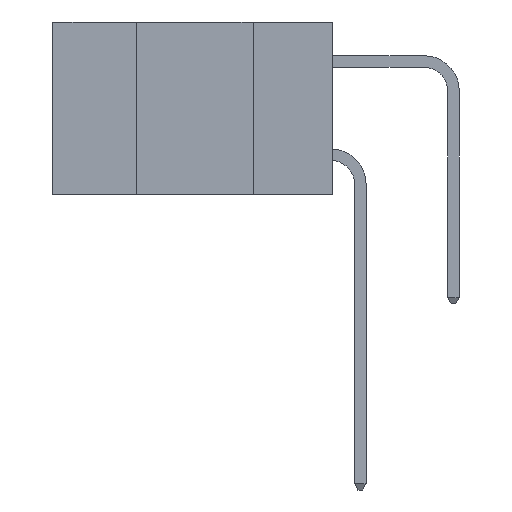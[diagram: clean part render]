
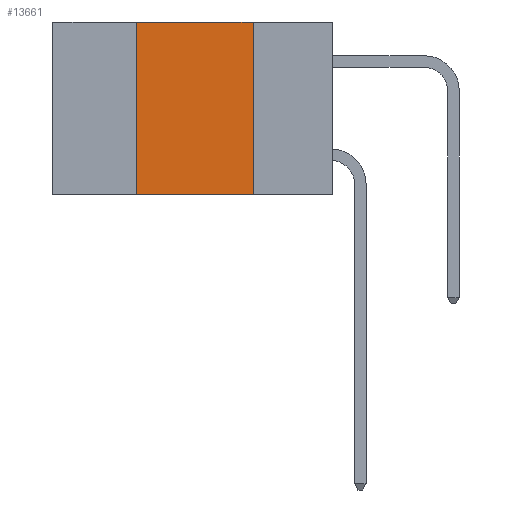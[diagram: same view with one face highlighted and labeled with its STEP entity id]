
A CAD part, left-side view. The second image highlights one B-rep face of the part: STEP entity #13661.
In plain terms, the highlighted planar face has unit normal (-1, 0, 0).
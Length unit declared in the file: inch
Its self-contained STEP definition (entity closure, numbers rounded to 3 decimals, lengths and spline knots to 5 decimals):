
#163 = EDGE_CURVE ( 'NONE', #5207, #4817, #5911, .T. ) ;
#889 = ORIENTED_EDGE ( 'NONE', *, *, #163, .F. ) ;
#1049 = CARTESIAN_POINT ( 'NONE',  ( 0., 0.42, -0.37 ) ) ;
#1085 = CARTESIAN_POINT ( 'NONE',  ( 0., 0.17, 0. ) ) ;
#1597 = VECTOR ( 'NONE', #5362, 39.37008 ) ;
#3284 = LINE ( 'NONE', #1049, #13535 ) ;
#3338 = EDGE_CURVE ( 'NONE', #12885, #10371, #3284, .T. ) ;
#3356 = VECTOR ( 'NONE', #5294, 39.37008 ) ;
#3458 = PLANE ( 'NONE',  #11560 ) ;
#4817 = VERTEX_POINT ( 'NONE', #5632 ) ;
#4936 = EDGE_LOOP ( 'NONE', ( #889, #6750, #7741, #13326 ) ) ;
#5207 = VERTEX_POINT ( 'NONE', #1085 ) ;
#5246 = EDGE_CURVE ( 'NONE', #10371, #5207, #6212, .T. ) ;
#5294 = DIRECTION ( 'NONE',  ( 0., -1., 0. ) ) ;
#5362 = DIRECTION ( 'NONE',  ( 0., -1., 0. ) ) ;
#5582 = VECTOR ( 'NONE', #8858, 39.37008 ) ;
#5632 = CARTESIAN_POINT ( 'NONE',  ( 0., 0.17, -0.37 ) ) ;
#5638 = DIRECTION ( 'NONE',  ( 0., 0., -1. ) ) ;
#5911 = LINE ( 'NONE', #10120, #5582 ) ;
#6212 = LINE ( 'NONE', #7506, #3356 ) ;
#6750 = ORIENTED_EDGE ( 'NONE', *, *, #5246, .F. ) ;
#7426 = DIRECTION ( 'NONE',  ( 0., 0., 1. ) ) ;
#7506 = CARTESIAN_POINT ( 'NONE',  ( 0., 0.6, 0. ) ) ;
#7741 = ORIENTED_EDGE ( 'NONE', *, *, #3338, .F. ) ;
#8436 = FACE_OUTER_BOUND ( 'NONE', #4936, .T. ) ;
#8858 = DIRECTION ( 'NONE',  ( 0., 0., -1. ) ) ;
#10102 = LINE ( 'NONE', #11674, #1597 ) ;
#10120 = CARTESIAN_POINT ( 'NONE',  ( 0., 0.17, -0.37 ) ) ;
#10371 = VERTEX_POINT ( 'NONE', #13054 ) ;
#10911 = CARTESIAN_POINT ( 'NONE',  ( 0., 0.6, 0. ) ) ;
#11560 = AXIS2_PLACEMENT_3D ( 'NONE', #10911, #11940, #5638 ) ;
#11674 = CARTESIAN_POINT ( 'NONE',  ( 0., 0.6, -0.37 ) ) ;
#11692 = CARTESIAN_POINT ( 'NONE',  ( 0., 0.42, -0.37 ) ) ;
#11940 = DIRECTION ( 'NONE',  ( 1., 0., 0. ) ) ;
#12885 = VERTEX_POINT ( 'NONE', #11692 ) ;
#13054 = CARTESIAN_POINT ( 'NONE',  ( 0., 0.42, 0. ) ) ;
#13326 = ORIENTED_EDGE ( 'NONE', *, *, #13521, .T. ) ;
#13521 = EDGE_CURVE ( 'NONE', #12885, #4817, #10102, .T. ) ;
#13535 = VECTOR ( 'NONE', #7426, 39.37008 ) ;
#13661 = ADVANCED_FACE ( 'NONE', ( #8436 ), #3458, .F. ) ;
